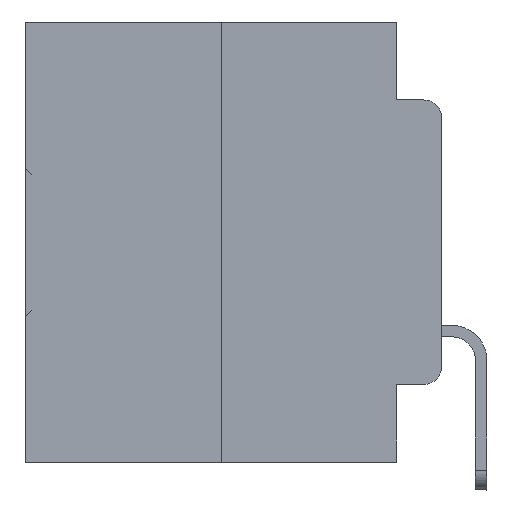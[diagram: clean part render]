
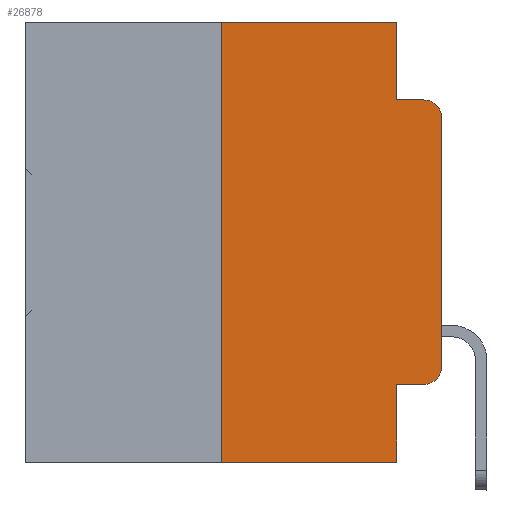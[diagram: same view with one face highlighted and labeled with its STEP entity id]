
A CAD part, left-side view. The second image highlights one B-rep face of the part: STEP entity #26878.
In plain terms, the highlighted planar face has unit normal (-1, 0, 0).
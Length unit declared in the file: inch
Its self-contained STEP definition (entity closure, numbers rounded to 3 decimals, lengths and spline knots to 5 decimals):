
#200 = VERTEX_POINT ( 'NONE', #17630 ) ;
#1143 = ORIENTED_EDGE ( 'NONE', *, *, #18680, .F. ) ;
#1738 = EDGE_CURVE ( 'NONE', #19025, #12668, #14605, .T. ) ;
#2208 = CARTESIAN_POINT ( 'NONE',  ( 0., 0., 0. ) ) ;
#2264 = ORIENTED_EDGE ( 'NONE', *, *, #27608, .F. ) ;
#2325 = DIRECTION ( 'NONE',  ( 0., 0., 1. ) ) ;
#2921 = EDGE_CURVE ( 'NONE', #26772, #11279, #25965, .T. ) ;
#3484 = CIRCLE ( 'NONE', #9498, 0.02 ) ;
#4102 = CARTESIAN_POINT ( 'NONE',  ( 0., 0., -0.1085 ) ) ;
#4126 = DIRECTION ( 'NONE',  ( 0., 0., -1. ) ) ;
#4186 = DIRECTION ( 'NONE',  ( 0., 0., 1. ) ) ;
#4824 = DIRECTION ( 'NONE',  ( 0., -1., 0. ) ) ;
#5569 = DIRECTION ( 'NONE',  ( 0., 0., -1. ) ) ;
#5911 = VECTOR ( 'NONE', #20385, 39.37008 ) ;
#6712 = CARTESIAN_POINT ( 'NONE',  ( 0., 0.051, 0. ) ) ;
#6977 = LINE ( 'NONE', #16844, #24587 ) ;
#6999 = CARTESIAN_POINT ( 'NONE',  ( 0., 0.473, 0. ) ) ;
#7032 = ORIENTED_EDGE ( 'NONE', *, *, #25582, .T. ) ;
#7656 = CARTESIAN_POINT ( 'NONE',  ( 0., 0.051, -0.4115 ) ) ;
#8337 = AXIS2_PLACEMENT_3D ( 'NONE', #8762, #19347, #8641 ) ;
#8641 = DIRECTION ( 'NONE',  ( 0., 0., -1. ) ) ;
#8762 = CARTESIAN_POINT ( 'NONE',  ( 0., 0.02, -0.1085 ) ) ;
#8974 = CARTESIAN_POINT ( 'NONE',  ( 0., 0.051, -0.0885 ) ) ;
#9286 = VERTEX_POINT ( 'NONE', #24417 ) ;
#9498 = AXIS2_PLACEMENT_3D ( 'NONE', #19613, #19842, #4126 ) ;
#9827 = CARTESIAN_POINT ( 'NONE',  ( 0., 0.051, -0.0885 ) ) ;
#10435 = VECTOR ( 'NONE', #4824, 39.37008 ) ;
#11279 = VERTEX_POINT ( 'NONE', #14091 ) ;
#11529 = LINE ( 'NONE', #6712, #20163 ) ;
#11876 = VECTOR ( 'NONE', #4186, 39.37008 ) ;
#12034 = VECTOR ( 'NONE', #12648, 39.37008 ) ;
#12648 = DIRECTION ( 'NONE',  ( 0., -1., 0. ) ) ;
#12668 = VERTEX_POINT ( 'NONE', #19054 ) ;
#13273 = LINE ( 'NONE', #7656, #10435 ) ;
#14091 = CARTESIAN_POINT ( 'NONE',  ( 0., 0.051, -0.5 ) ) ;
#14605 = LINE ( 'NONE', #9827, #5911 ) ;
#14803 = EDGE_CURVE ( 'NONE', #26772, #9286, #27003, .T. ) ;
#14948 = VECTOR ( 'NONE', #2325, 39.37008 ) ;
#15076 = VERTEX_POINT ( 'NONE', #31527 ) ;
#15425 = VECTOR ( 'NONE', #22607, 39.37008 ) ;
#15535 = ORIENTED_EDGE ( 'NONE', *, *, #14803, .F. ) ;
#16005 = VERTEX_POINT ( 'NONE', #4102 ) ;
#16294 = ORIENTED_EDGE ( 'NONE', *, *, #25577, .T. ) ;
#16298 = ORIENTED_EDGE ( 'NONE', *, *, #20684, .T. ) ;
#16844 = CARTESIAN_POINT ( 'NONE',  ( 0., 0.051, 0. ) ) ;
#17284 = CARTESIAN_POINT ( 'NONE',  ( 0., 0.25, 0. ) ) ;
#17527 = DIRECTION ( 'NONE',  ( 0., 0., -1. ) ) ;
#17630 = CARTESIAN_POINT ( 'NONE',  ( 0., 0.02, -0.4115 ) ) ;
#18680 = EDGE_CURVE ( 'NONE', #25284, #11279, #6977, .T. ) ;
#19025 = VERTEX_POINT ( 'NONE', #8974 ) ;
#19054 = CARTESIAN_POINT ( 'NONE',  ( 0., 0.02, -0.0885 ) ) ;
#19347 = DIRECTION ( 'NONE',  ( -1., 0., 0. ) ) ;
#19613 = CARTESIAN_POINT ( 'NONE',  ( 0., 0.02, -0.3915 ) ) ;
#19842 = DIRECTION ( 'NONE',  ( -1., 0., 0. ) ) ;
#20163 = VECTOR ( 'NONE', #28486, 39.37008 ) ;
#20385 = DIRECTION ( 'NONE',  ( 0., -1., 0. ) ) ;
#20684 = EDGE_CURVE ( 'NONE', #16005, #12668, #23651, .T. ) ;
#21501 = DIRECTION ( 'NONE',  ( 1., 0., 0. ) ) ;
#22390 = LINE ( 'NONE', #6999, #15425 ) ;
#22607 = DIRECTION ( 'NONE',  ( 0., -1., 0. ) ) ;
#23651 = CIRCLE ( 'NONE', #8337, 0.02 ) ;
#23738 = CARTESIAN_POINT ( 'NONE',  ( 0., 0.051, -0.4115 ) ) ;
#23746 = ORIENTED_EDGE ( 'NONE', *, *, #2921, .T. ) ;
#24417 = CARTESIAN_POINT ( 'NONE',  ( 0., 0.25, 0. ) ) ;
#24587 = VECTOR ( 'NONE', #17527, 39.37008 ) ;
#24740 = AXIS2_PLACEMENT_3D ( 'NONE', #33804, #21501, #5569 ) ;
#24756 = EDGE_LOOP ( 'NONE', ( #16294, #16298, #25725, #2264, #28574, #15535, #23746, #1143, #7032, #32502 ) ) ;
#25284 = VERTEX_POINT ( 'NONE', #23738 ) ;
#25577 = EDGE_CURVE ( 'NONE', #25959, #16005, #27214, .T. ) ;
#25582 = EDGE_CURVE ( 'NONE', #25284, #200, #13273, .T. ) ;
#25725 = ORIENTED_EDGE ( 'NONE', *, *, #1738, .F. ) ;
#25929 = FACE_OUTER_BOUND ( 'NONE', #24756, .T. ) ;
#25959 = VERTEX_POINT ( 'NONE', #26883 ) ;
#25965 = LINE ( 'NONE', #33834, #12034 ) ;
#26772 = VERTEX_POINT ( 'NONE', #33687 ) ;
#26878 = ADVANCED_FACE ( 'NONE', ( #25929 ), #33696, .F. ) ;
#26883 = CARTESIAN_POINT ( 'NONE',  ( 0., 0., -0.3915 ) ) ;
#27003 = LINE ( 'NONE', #17284, #11876 ) ;
#27214 = LINE ( 'NONE', #2208, #14948 ) ;
#27608 = EDGE_CURVE ( 'NONE', #15076, #19025, #11529, .T. ) ;
#28486 = DIRECTION ( 'NONE',  ( 0., 0., -1. ) ) ;
#28574 = ORIENTED_EDGE ( 'NONE', *, *, #30835, .F. ) ;
#30835 = EDGE_CURVE ( 'NONE', #9286, #15076, #22390, .T. ) ;
#31527 = CARTESIAN_POINT ( 'NONE',  ( 0., 0.051, 0. ) ) ;
#31891 = EDGE_CURVE ( 'NONE', #200, #25959, #3484, .T. ) ;
#32502 = ORIENTED_EDGE ( 'NONE', *, *, #31891, .T. ) ;
#33687 = CARTESIAN_POINT ( 'NONE',  ( 0., 0.25, -0.5 ) ) ;
#33696 = PLANE ( 'NONE',  #24740 ) ;
#33804 = CARTESIAN_POINT ( 'NONE',  ( 0., 0.473, 0. ) ) ;
#33834 = CARTESIAN_POINT ( 'NONE',  ( 0., 0.473, -0.5 ) ) ;
